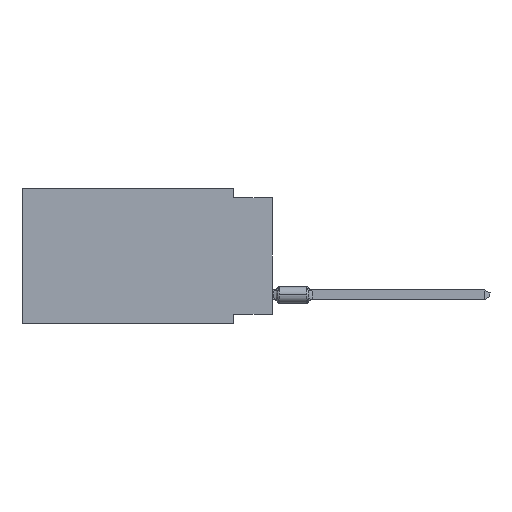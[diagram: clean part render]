
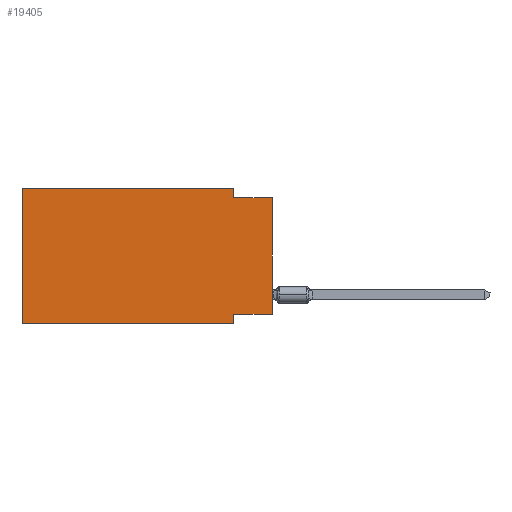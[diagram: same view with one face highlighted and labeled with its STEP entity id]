
A CAD part, left-side view. The second image highlights one B-rep face of the part: STEP entity #19405.
In plain terms, the highlighted planar face has unit normal (-1, 0, 0).
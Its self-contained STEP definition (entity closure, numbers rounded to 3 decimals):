
#957 = AXIS2_PLACEMENT_3D ( 'NONE', #55098, #13116, #21860 ) ;
#1116 = VECTOR ( 'NONE', #21327, 1000. ) ;
#3587 = VERTEX_POINT ( 'NONE', #41223 ) ;
#3820 = CARTESIAN_POINT ( 'NONE',  ( 0., 2.54, -8.255 ) ) ;
#6706 = DIRECTION ( 'NONE',  ( 0., 0., -1. ) ) ;
#6811 = LINE ( 'NONE', #7082, #19925 ) ;
#7082 = CARTESIAN_POINT ( 'NONE',  ( 0., 2.54, 0. ) ) ;
#8365 = ORIENTED_EDGE ( 'NONE', *, *, #33346, .F. ) ;
#8992 = CARTESIAN_POINT ( 'NONE',  ( 0., 16.383, 0. ) ) ;
#10213 = DIRECTION ( 'NONE',  ( 0., 0., -1. ) ) ;
#10376 = DIRECTION ( 'NONE',  ( 0., -1., 0. ) ) ;
#11662 = VECTOR ( 'NONE', #10376, 1000. ) ;
#12147 = DIRECTION ( 'NONE',  ( 0., 0., 1. ) ) ;
#12187 = LINE ( 'NONE', #34174, #32721 ) ;
#12547 = FACE_OUTER_BOUND ( 'NONE', #31662, .T. ) ;
#13116 = DIRECTION ( 'NONE',  ( 1., 0., 0. ) ) ;
#13203 = VERTEX_POINT ( 'NONE', #31303 ) ;
#13805 = VECTOR ( 'NONE', #12147, 1000. ) ;
#14470 = ORIENTED_EDGE ( 'NONE', *, *, #43523, .F. ) ;
#14631 = CARTESIAN_POINT ( 'NONE',  ( 0., 2.54, -8.89 ) ) ;
#15445 = EDGE_CURVE ( 'NONE', #43899, #44797, #18609, .T. ) ;
#17027 = ORIENTED_EDGE ( 'NONE', *, *, #15445, .F. ) ;
#18609 = LINE ( 'NONE', #35783, #22417 ) ;
#19405 = ADVANCED_FACE ( 'NONE', ( #12547 ), #29740, .F. ) ;
#19925 = VECTOR ( 'NONE', #10213, 1000. ) ;
#20599 = EDGE_CURVE ( 'NONE', #53200, #26715, #12187, .T. ) ;
#21054 = LINE ( 'NONE', #50892, #1116 ) ;
#21078 = CARTESIAN_POINT ( 'NONE',  ( 0., 2.54, 0. ) ) ;
#21327 = DIRECTION ( 'NONE',  ( 0., -1., 0. ) ) ;
#21860 = DIRECTION ( 'NONE',  ( 0., 0., -1. ) ) ;
#22417 = VECTOR ( 'NONE', #52678, 1000. ) ;
#22523 = VECTOR ( 'NONE', #6706, 1000. ) ;
#23382 = CARTESIAN_POINT ( 'NONE',  ( 0., 0., -8.255 ) ) ;
#24898 = DIRECTION ( 'NONE',  ( 0., 1., 0. ) ) ;
#26715 = VERTEX_POINT ( 'NONE', #3820 ) ;
#29740 = PLANE ( 'NONE',  #957 ) ;
#31303 = CARTESIAN_POINT ( 'NONE',  ( 0., 2.54, -8.89 ) ) ;
#31662 = EDGE_LOOP ( 'NONE', ( #46925, #37696, #14470, #39396, #17027, #43807, #8365, #44641 ) ) ;
#32097 = LINE ( 'NONE', #53218, #11662 ) ;
#32721 = VECTOR ( 'NONE', #24898, 1000. ) ;
#33346 = EDGE_CURVE ( 'NONE', #26715, #13203, #36327, .T. ) ;
#33392 = EDGE_CURVE ( 'NONE', #43899, #13203, #32097, .T. ) ;
#34174 = CARTESIAN_POINT ( 'NONE',  ( 0., 0., -8.255 ) ) ;
#34212 = VERTEX_POINT ( 'NONE', #37404 ) ;
#34969 = VERTEX_POINT ( 'NONE', #21078 ) ;
#35783 = CARTESIAN_POINT ( 'NONE',  ( 0., 16.383, 0. ) ) ;
#35873 = EDGE_CURVE ( 'NONE', #44797, #34969, #52649, .T. ) ;
#36327 = LINE ( 'NONE', #14631, #22523 ) ;
#36750 = CARTESIAN_POINT ( 'NONE',  ( 0., 16.383, -8.89 ) ) ;
#37404 = CARTESIAN_POINT ( 'NONE',  ( 0., 2.54, -0.635 ) ) ;
#37696 = ORIENTED_EDGE ( 'NONE', *, *, #44711, .F. ) ;
#39321 = CARTESIAN_POINT ( 'NONE',  ( 0., 16.383, 0. ) ) ;
#39396 = ORIENTED_EDGE ( 'NONE', *, *, #35873, .F. ) ;
#41223 = CARTESIAN_POINT ( 'NONE',  ( 0., 0., -0.635 ) ) ;
#43523 = EDGE_CURVE ( 'NONE', #34969, #34212, #6811, .T. ) ;
#43807 = ORIENTED_EDGE ( 'NONE', *, *, #33392, .T. ) ;
#43899 = VERTEX_POINT ( 'NONE', #36750 ) ;
#44204 = DIRECTION ( 'NONE',  ( 0., -1., 0. ) ) ;
#44641 = ORIENTED_EDGE ( 'NONE', *, *, #20599, .F. ) ;
#44711 = EDGE_CURVE ( 'NONE', #34212, #3587, #21054, .T. ) ;
#44797 = VERTEX_POINT ( 'NONE', #39321 ) ;
#45504 = EDGE_CURVE ( 'NONE', #53200, #3587, #46515, .T. ) ;
#46515 = LINE ( 'NONE', #54138, #13805 ) ;
#46925 = ORIENTED_EDGE ( 'NONE', *, *, #45504, .T. ) ;
#50485 = VECTOR ( 'NONE', #44204, 1000. ) ;
#50892 = CARTESIAN_POINT ( 'NONE',  ( 0., 0., -0.635 ) ) ;
#52649 = LINE ( 'NONE', #8992, #50485 ) ;
#52678 = DIRECTION ( 'NONE',  ( 0., 0., 1. ) ) ;
#53200 = VERTEX_POINT ( 'NONE', #23382 ) ;
#53218 = CARTESIAN_POINT ( 'NONE',  ( 0., 16.383, -8.89 ) ) ;
#54138 = CARTESIAN_POINT ( 'NONE',  ( 0., 0., 0. ) ) ;
#55098 = CARTESIAN_POINT ( 'NONE',  ( 0., 16.383, 0. ) ) ;
